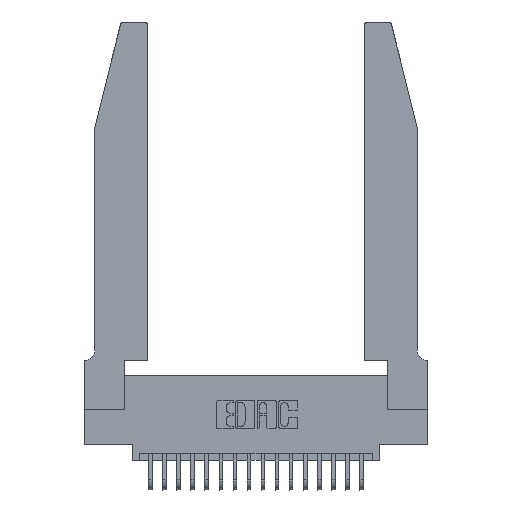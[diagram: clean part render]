
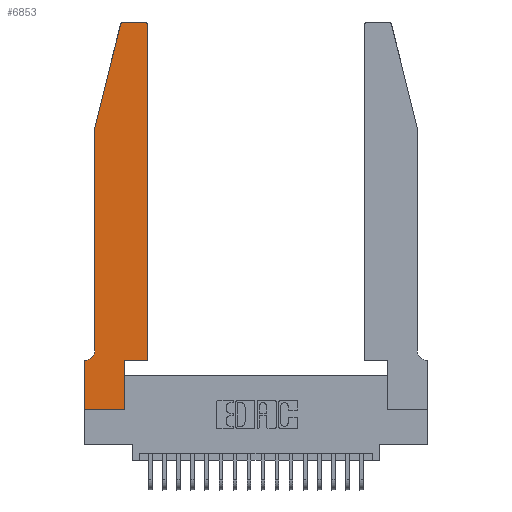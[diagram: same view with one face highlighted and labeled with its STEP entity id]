
A CAD part, top view. The second image highlights one B-rep face of the part: STEP entity #6853.
In plain terms, the highlighted planar face has unit normal (0, 0, 1).
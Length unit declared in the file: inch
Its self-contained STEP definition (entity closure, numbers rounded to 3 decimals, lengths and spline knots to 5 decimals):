
#317 = DIRECTION ( 'NONE',  ( 0., 0., 1. ) ) ;
#324 = VECTOR ( 'NONE', #18339, 39.37008 ) ;
#772 = VECTOR ( 'NONE', #16814, 39.37008 ) ;
#973 = CARTESIAN_POINT ( 'NONE',  ( 0.4505, 0.35, 0.37 ) ) ;
#983 = ORIENTED_EDGE ( 'NONE', *, *, #4632, .T. ) ;
#1060 = PLANE ( 'NONE',  #19540 ) ;
#1169 = VERTEX_POINT ( 'NONE', #18174 ) ;
#1370 = VECTOR ( 'NONE', #15183, 39.37008 ) ;
#1638 = CARTESIAN_POINT ( 'NONE',  ( 0., 0.35, 0.37 ) ) ;
#1828 = DIRECTION ( 'NONE',  ( -1., 0., 0. ) ) ;
#1875 = EDGE_CURVE ( 'NONE', #8164, #7098, #9814, .T. ) ;
#1955 = LINE ( 'NONE', #13518, #1370 ) ;
#2012 = ORIENTED_EDGE ( 'NONE', *, *, #8002, .T. ) ;
#2183 = DIRECTION ( 'NONE',  ( 1., 0., 0. ) ) ;
#2457 = EDGE_CURVE ( 'NONE', #7073, #16880, #5572, .T. ) ;
#2504 = ORIENTED_EDGE ( 'NONE', *, *, #1875, .T. ) ;
#2953 = DIRECTION ( 'NONE',  ( 0., 0., 1. ) ) ;
#3152 = CARTESIAN_POINT ( 'NONE',  ( 0.284, 2.72, 0.37 ) ) ;
#3177 = EDGE_LOOP ( 'NONE', ( #8075, #21547, #19973, #13476, #22623, #6640, #8691, #2012, #7023, #2504, #3544, #983 ) ) ;
#3544 = ORIENTED_EDGE ( 'NONE', *, *, #17340, .T. ) ;
#3612 = AXIS2_PLACEMENT_3D ( 'NONE', #11153, #317, #12859 ) ;
#3891 = VERTEX_POINT ( 'NONE', #17164 ) ;
#4198 = CARTESIAN_POINT ( 'NONE',  ( 0.25487, 2.72718, 0.37 ) ) ;
#4632 = EDGE_CURVE ( 'NONE', #5035, #3891, #9511, .T. ) ;
#4682 = DIRECTION ( 'NONE',  ( 0., -1., 0. ) ) ;
#4728 = CARTESIAN_POINT ( 'NONE',  ( 0., 0., 0.37 ) ) ;
#4944 = DIRECTION ( 'NONE',  ( 1., 0., 0. ) ) ;
#5035 = VERTEX_POINT ( 'NONE', #13758 ) ;
#5135 = VECTOR ( 'NONE', #1828, 39.37008 ) ;
#5347 = CIRCLE ( 'NONE', #20615, 0.07 ) ;
#5572 = LINE ( 'NONE', #4728, #18725 ) ;
#5654 = DIRECTION ( 'NONE',  ( 0., 0., -1. ) ) ;
#6357 = CARTESIAN_POINT ( 'NONE',  ( 0.4505, 0.35, 0.37 ) ) ;
#6640 = ORIENTED_EDGE ( 'NONE', *, *, #17612, .T. ) ;
#6853 = ADVANCED_FACE ( 'NONE', ( #13711 ), #1060, .T. ) ;
#6868 = LINE ( 'NONE', #20049, #15469 ) ;
#6938 = VERTEX_POINT ( 'NONE', #16979 ) ;
#7023 = ORIENTED_EDGE ( 'NONE', *, *, #22031, .T. ) ;
#7073 = VERTEX_POINT ( 'NONE', #1638 ) ;
#7098 = VERTEX_POINT ( 'NONE', #12453 ) ;
#7424 = EDGE_CURVE ( 'NONE', #19964, #19518, #8587, .T. ) ;
#8002 = EDGE_CURVE ( 'NONE', #16880, #6938, #6868, .T. ) ;
#8075 = ORIENTED_EDGE ( 'NONE', *, *, #14473, .T. ) ;
#8164 = VERTEX_POINT ( 'NONE', #22286 ) ;
#8587 = CIRCLE ( 'NONE', #11998, 0.03 ) ;
#8646 = VECTOR ( 'NONE', #15910, 39.37008 ) ;
#8691 = ORIENTED_EDGE ( 'NONE', *, *, #2457, .T. ) ;
#9115 = CARTESIAN_POINT ( 'NONE',  ( 0.0755, 0.42, 0.37 ) ) ;
#9511 = CIRCLE ( 'NONE', #3612, 0.03 ) ;
#9725 = EDGE_CURVE ( 'NONE', #19518, #1169, #9873, .T. ) ;
#9814 = LINE ( 'NONE', #973, #13836 ) ;
#9873 = LINE ( 'NONE', #21948, #772 ) ;
#9928 = EDGE_CURVE ( 'NONE', #12653, #17181, #5347, .T. ) ;
#10106 = VECTOR ( 'NONE', #14128, 39.37008 ) ;
#10692 = CARTESIAN_POINT ( 'NONE',  ( 0.2865, 0.35, 0.37 ) ) ;
#11153 = CARTESIAN_POINT ( 'NONE',  ( 0.4205, 2.72, 0.37 ) ) ;
#11453 = CARTESIAN_POINT ( 'NONE',  ( 0., 0., 0.37 ) ) ;
#11998 = AXIS2_PLACEMENT_3D ( 'NONE', #3152, #15393, #4944 ) ;
#12453 = CARTESIAN_POINT ( 'NONE',  ( 0.4505, 0.35, 0.37 ) ) ;
#12474 = CARTESIAN_POINT ( 'NONE',  ( 0.2605, 2.75, 0.37 ) ) ;
#12653 = VERTEX_POINT ( 'NONE', #9115 ) ;
#12859 = DIRECTION ( 'NONE',  ( 1., 0., 0. ) ) ;
#13476 = ORIENTED_EDGE ( 'NONE', *, *, #15718, .T. ) ;
#13518 = CARTESIAN_POINT ( 'NONE',  ( 0.0755, 2., 0.37 ) ) ;
#13711 = FACE_OUTER_BOUND ( 'NONE', #3177, .T. ) ;
#13758 = CARTESIAN_POINT ( 'NONE',  ( 0.4505, 2.72, 0.37 ) ) ;
#13836 = VECTOR ( 'NONE', #2183, 39.37008 ) ;
#14128 = DIRECTION ( 'NONE',  ( 0., 1., 0. ) ) ;
#14292 = CARTESIAN_POINT ( 'NONE',  ( 0.0755, 0.35, 0.37 ) ) ;
#14472 = LINE ( 'NONE', #12474, #5135 ) ;
#14473 = EDGE_CURVE ( 'NONE', #3891, #19964, #14472, .T. ) ;
#14555 = LINE ( 'NONE', #6357, #324 ) ;
#15183 = DIRECTION ( 'NONE',  ( 0., -1., 0. ) ) ;
#15208 = DIRECTION ( 'NONE',  ( 1., 0., 0. ) ) ;
#15393 = DIRECTION ( 'NONE',  ( 0., 0., 1. ) ) ;
#15469 = VECTOR ( 'NONE', #20121, 39.37008 ) ;
#15718 = EDGE_CURVE ( 'NONE', #1169, #12653, #1955, .T. ) ;
#15910 = DIRECTION ( 'NONE',  ( -1., 0., 0. ) ) ;
#16006 = CARTESIAN_POINT ( 'NONE',  ( 0.0055, 0.42, 0.37 ) ) ;
#16767 = CARTESIAN_POINT ( 'NONE',  ( 0., 0.35, 0.37 ) ) ;
#16814 = DIRECTION ( 'NONE',  ( -0.239, -0.971, 0. ) ) ;
#16880 = VERTEX_POINT ( 'NONE', #11453 ) ;
#16979 = CARTESIAN_POINT ( 'NONE',  ( 0.2865, 0., 0.37 ) ) ;
#17164 = CARTESIAN_POINT ( 'NONE',  ( 0.4205, 2.75, 0.37 ) ) ;
#17181 = VERTEX_POINT ( 'NONE', #17671 ) ;
#17340 = EDGE_CURVE ( 'NONE', #7098, #5035, #14555, .T. ) ;
#17612 = EDGE_CURVE ( 'NONE', #17181, #7073, #22154, .T. ) ;
#17651 = DIRECTION ( 'NONE',  ( -1., 0., 0. ) ) ;
#17671 = CARTESIAN_POINT ( 'NONE',  ( 0.0055, 0.35, 0.37 ) ) ;
#18174 = CARTESIAN_POINT ( 'NONE',  ( 0.0755, 2., 0.37 ) ) ;
#18339 = DIRECTION ( 'NONE',  ( 0., 1., 0. ) ) ;
#18725 = VECTOR ( 'NONE', #4682, 39.37008 ) ;
#19011 = LINE ( 'NONE', #10692, #10106 ) ;
#19105 = CARTESIAN_POINT ( 'NONE',  ( 0.284, 2.75, 0.37 ) ) ;
#19518 = VERTEX_POINT ( 'NONE', #4198 ) ;
#19540 = AXIS2_PLACEMENT_3D ( 'NONE', #16767, #2953, #15208 ) ;
#19964 = VERTEX_POINT ( 'NONE', #19105 ) ;
#19973 = ORIENTED_EDGE ( 'NONE', *, *, #9725, .T. ) ;
#20049 = CARTESIAN_POINT ( 'NONE',  ( 0., 0., 0.37 ) ) ;
#20121 = DIRECTION ( 'NONE',  ( 1., 0., 0. ) ) ;
#20615 = AXIS2_PLACEMENT_3D ( 'NONE', #16006, #5654, #17651 ) ;
#21547 = ORIENTED_EDGE ( 'NONE', *, *, #7424, .T. ) ;
#21948 = CARTESIAN_POINT ( 'NONE',  ( 0.0755, 2., 0.37 ) ) ;
#22031 = EDGE_CURVE ( 'NONE', #6938, #8164, #19011, .T. ) ;
#22154 = LINE ( 'NONE', #14292, #8646 ) ;
#22286 = CARTESIAN_POINT ( 'NONE',  ( 0.2865, 0.35, 0.37 ) ) ;
#22623 = ORIENTED_EDGE ( 'NONE', *, *, #9928, .T. ) ;
